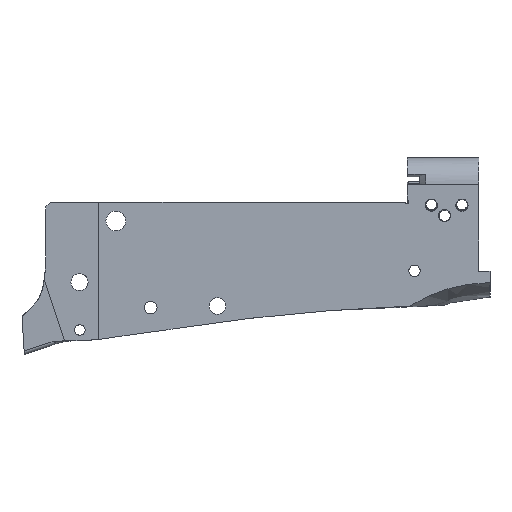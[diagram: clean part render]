
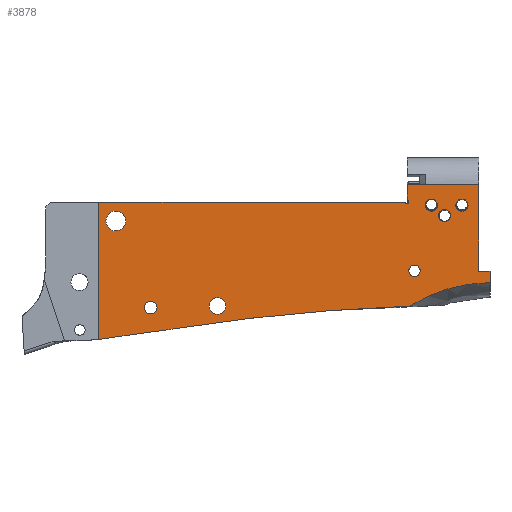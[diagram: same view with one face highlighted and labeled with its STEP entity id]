
A CAD part, left-side view. The second image highlights one B-rep face of the part: STEP entity #3878.
In plain terms, the highlighted planar face has unit normal (-1, 0, 0).
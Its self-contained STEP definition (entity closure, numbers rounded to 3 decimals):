
#116=FACE_BOUND('',#637,.T.);
#117=FACE_BOUND('',#638,.T.);
#118=FACE_BOUND('',#639,.T.);
#119=FACE_BOUND('',#640,.T.);
#120=FACE_BOUND('',#641,.T.);
#121=FACE_BOUND('',#642,.T.);
#122=FACE_BOUND('',#643,.T.);
#223=PLANE('',#4232);
#405=FACE_OUTER_BOUND('',#636,.T.);
#636=EDGE_LOOP('',(#3380,#3381,#3382,#3383,#3384,#3385,#3386,#3387,#3388,
#3389,#3390,#3391,#3392,#3393,#3394));
#637=EDGE_LOOP('',(#3395));
#638=EDGE_LOOP('',(#3396));
#639=EDGE_LOOP('',(#3397));
#640=EDGE_LOOP('',(#3398));
#641=EDGE_LOOP('',(#3399));
#642=EDGE_LOOP('',(#3400));
#643=EDGE_LOOP('',(#3401));
#865=LINE('',#6095,#1246);
#928=LINE('',#6402,#1309);
#962=LINE('',#6740,#1343);
#964=LINE('',#6747,#1345);
#965=LINE('',#6750,#1346);
#992=LINE('',#6824,#1373);
#1018=LINE('',#7119,#1399);
#1023=LINE('',#7130,#1404);
#1246=VECTOR('',#4724,10.);
#1309=VECTOR('',#4911,10.);
#1343=VECTOR('',#5021,10.);
#1345=VECTOR('',#5029,10.);
#1346=VECTOR('',#5034,10.);
#1373=VECTOR('',#5117,10.);
#1399=VECTOR('',#5197,10.);
#1404=VECTOR('',#5210,10.);
#1459=CIRCLE('',#3940,100.);
#1477=CIRCLE('',#3960,827.021);
#1498=CIRCLE('',#3984,600.987);
#1501=CIRCLE('',#3987,45.79);
#1521=CIRCLE('',#4055,1.85);
#1522=CIRCLE('',#4056,1.85);
#1523=CIRCLE('',#4058,1.85);
#1524=CIRCLE('',#4062,2.5);
#1572=CIRCLE('',#4181,3.);
#1573=CIRCLE('',#4184,1.9);
#1587=CIRCLE('',#4231,0.5);
#1588=CIRCLE('',#4233,0.5);
#1589=CIRCLE('',#4234,0.5);
#1590=CIRCLE('',#4235,1.75);
#1601=VERTEX_POINT('',#5389);
#1602=VERTEX_POINT('',#5390);
#1636=VERTEX_POINT('',#5462);
#1667=VERTEX_POINT('',#5531);
#1669=VERTEX_POINT('',#5566);
#1781=VERTEX_POINT('',#5894);
#1783=VERTEX_POINT('',#5967);
#1785=VERTEX_POINT('',#6023);
#1787=VERTEX_POINT('',#6074);
#1792=VERTEX_POINT('',#6092);
#1793=VERTEX_POINT('',#6094);
#1864=VERTEX_POINT('',#6393);
#1867=VERTEX_POINT('',#6400);
#1903=VERTEX_POINT('',#6738);
#1905=VERTEX_POINT('',#6746);
#1909=VERTEX_POINT('',#6767);
#1910=VERTEX_POINT('',#6773);
#1924=VERTEX_POINT('',#6822);
#1942=VERTEX_POINT('',#7124);
#1943=VERTEX_POINT('',#7125);
#1944=VERTEX_POINT('',#7131);
#1945=VERTEX_POINT('',#7134);
#1970=EDGE_CURVE('',#1601,#1602,#1459,.T.);
#2006=EDGE_CURVE('',#1636,#1602,#1477,.T.);
#2042=EDGE_CURVE('',#1601,#1667,#1498,.T.);
#2045=EDGE_CURVE('',#1667,#1669,#1501,.T.);
#2198=EDGE_CURVE('',#1781,#1781,#1521,.T.);
#2201=EDGE_CURVE('',#1783,#1783,#1522,.T.);
#2205=EDGE_CURVE('',#1785,#1785,#1523,.T.);
#2209=EDGE_CURVE('',#1787,#1787,#1524,.T.);
#2219=EDGE_CURVE('',#1792,#1793,#865,.T.);
#2323=EDGE_CURVE('',#1864,#1867,#928,.F.);
#2381=EDGE_CURVE('',#1792,#1903,#962,.T.);
#2384=EDGE_CURVE('',#1793,#1905,#964,.T.);
#2386=EDGE_CURVE('',#1669,#1905,#965,.T.);
#2396=EDGE_CURVE('',#1909,#1909,#1572,.T.);
#2399=EDGE_CURVE('',#1910,#1910,#1573,.T.);
#2423=EDGE_CURVE('',#1924,#1903,#992,.T.);
#2461=EDGE_CURVE('',#1867,#1636,#1018,.T.);
#2464=EDGE_CURVE('',#1942,#1943,#1587,.T.);
#2467=EDGE_CURVE('',#1924,#1943,#1023,.F.);
#2468=EDGE_CURVE('',#1942,#1944,#1588,.T.);
#2469=EDGE_CURVE('',#1864,#1944,#1589,.T.);
#2470=EDGE_CURVE('',#1945,#1945,#1590,.T.);
#3380=ORIENTED_EDGE('',*,*,#1970,.F.);
#3381=ORIENTED_EDGE('',*,*,#2042,.T.);
#3382=ORIENTED_EDGE('',*,*,#2045,.T.);
#3383=ORIENTED_EDGE('',*,*,#2386,.T.);
#3384=ORIENTED_EDGE('',*,*,#2384,.F.);
#3385=ORIENTED_EDGE('',*,*,#2219,.F.);
#3386=ORIENTED_EDGE('',*,*,#2381,.T.);
#3387=ORIENTED_EDGE('',*,*,#2423,.F.);
#3388=ORIENTED_EDGE('',*,*,#2467,.T.);
#3389=ORIENTED_EDGE('',*,*,#2464,.F.);
#3390=ORIENTED_EDGE('',*,*,#2468,.T.);
#3391=ORIENTED_EDGE('',*,*,#2469,.F.);
#3392=ORIENTED_EDGE('',*,*,#2323,.T.);
#3393=ORIENTED_EDGE('',*,*,#2461,.T.);
#3394=ORIENTED_EDGE('',*,*,#2006,.T.);
#3395=ORIENTED_EDGE('',*,*,#2470,.T.);
#3396=ORIENTED_EDGE('',*,*,#2399,.T.);
#3397=ORIENTED_EDGE('',*,*,#2396,.T.);
#3398=ORIENTED_EDGE('',*,*,#2209,.T.);
#3399=ORIENTED_EDGE('',*,*,#2198,.T.);
#3400=ORIENTED_EDGE('',*,*,#2201,.T.);
#3401=ORIENTED_EDGE('',*,*,#2205,.T.);
#3878=ADVANCED_FACE('',(#405,#116,#117,#118,#119,#120,#121,#122),#223,.F.);
#3940=AXIS2_PLACEMENT_3D('',#5391,#4298,#4299);
#3960=AXIS2_PLACEMENT_3D('',#5463,#4356,#4357);
#3984=AXIS2_PLACEMENT_3D('',#5548,#4418,#4419);
#3987=AXIS2_PLACEMENT_3D('',#5568,#4424,#4425);
#4055=AXIS2_PLACEMENT_3D('',#5895,#4686,#4687);
#4056=AXIS2_PLACEMENT_3D('',#5968,#4688,#4689);
#4058=AXIS2_PLACEMENT_3D('',#6025,#4693,#4694);
#4062=AXIS2_PLACEMENT_3D('',#6075,#4703,#4704);
#4181=AXIS2_PLACEMENT_3D('',#6769,#5056,#5057);
#4184=AXIS2_PLACEMENT_3D('',#6775,#5064,#5065);
#4231=AXIS2_PLACEMENT_3D('',#7126,#5204,#5205);
#4232=AXIS2_PLACEMENT_3D('',#7129,#5208,#5209);
#4233=AXIS2_PLACEMENT_3D('',#7132,#5211,#5212);
#4234=AXIS2_PLACEMENT_3D('',#7133,#5213,#5214);
#4235=AXIS2_PLACEMENT_3D('',#7135,#5215,#5216);
#4298=DIRECTION('center_axis',(1.,0.,0.));
#4299=DIRECTION('ref_axis',(0.,-0.143,-0.99));
#4356=DIRECTION('center_axis',(1.,0.,0.));
#4357=DIRECTION('ref_axis',(0.,0.184,0.983));
#4418=DIRECTION('center_axis',(1.,0.,0.));
#4419=DIRECTION('ref_axis',(0.,0.157,0.988));
#4424=DIRECTION('center_axis',(1.,0.,0.));
#4425=DIRECTION('ref_axis',(0.,0.008,1.));
#4686=DIRECTION('center_axis',(1.,0.,0.));
#4687=DIRECTION('ref_axis',(0.,1.,0.));
#4688=DIRECTION('center_axis',(1.,0.,0.));
#4689=DIRECTION('ref_axis',(0.,1.,0.));
#4693=DIRECTION('center_axis',(1.,0.,0.));
#4694=DIRECTION('ref_axis',(0.,-1.,0.));
#4703=DIRECTION('center_axis',(1.,0.,0.));
#4704=DIRECTION('ref_axis',(0.,-1.,0.));
#4724=DIRECTION('',(0.,-1.,0.));
#4911=DIRECTION('',(0.,-1.,0.));
#5021=DIRECTION('',(0.,0.,1.));
#5029=DIRECTION('',(0.,0.,-1.));
#5034=DIRECTION('',(0.,-1.,0.));
#5056=DIRECTION('center_axis',(1.,0.,0.));
#5057=DIRECTION('ref_axis',(0.,1.,0.));
#5064=DIRECTION('center_axis',(1.,0.,0.));
#5065=DIRECTION('ref_axis',(0.,1.,0.));
#5117=DIRECTION('',(0.,-1.,0.));
#5197=DIRECTION('',(0.,0.,-1.));
#5204=DIRECTION('center_axis',(1.,0.,0.));
#5205=DIRECTION('ref_axis',(0.,0.866,-0.5));
#5208=DIRECTION('center_axis',(1.,0.,0.));
#5209=DIRECTION('ref_axis',(0.,1.,0.));
#5210=DIRECTION('',(0.,0.,1.));
#5211=DIRECTION('center_axis',(1.,0.,0.));
#5212=DIRECTION('ref_axis',(0.,1.,0.));
#5213=DIRECTION('center_axis',(1.,0.,0.));
#5214=DIRECTION('ref_axis',(0.,-0.5,0.866));
#5215=DIRECTION('center_axis',(1.,0.,0.));
#5216=DIRECTION('ref_axis',(0.,1.,0.));
#5389=CARTESIAN_POINT('',(-16.48,94.298,-0.025));
#5390=CARTESIAN_POINT('',(-16.48,96.799,-0.385));
#5391=CARTESIAN_POINT('Origin',(-16.48,109.817,98.764));
#5462=CARTESIAN_POINT('',(-16.48,116.868,-3.271));
#5463=CARTESIAN_POINT('Origin',(-16.48,-10.864,-820.368));
#5531=CARTESIAN_POINT('',(-16.48,22.637,6.867));
#5548=CARTESIAN_POINT('Origin',(-16.48,1.034,-593.732));
#5566=CARTESIAN_POINT('',(-16.48,-1.532,13.989));
#5568=CARTESIAN_POINT('Origin',(-16.48,-1.889,-31.8));
#5894=CARTESIAN_POINT('',(-16.48,14.268,37.491));
#5895=CARTESIAN_POINT('Origin',(-16.48,16.118,37.491));
#5967=CARTESIAN_POINT('',(-16.48,4.968,37.491));
#5968=CARTESIAN_POINT('Origin',(-16.48,6.818,37.491));
#6023=CARTESIAN_POINT('',(-16.48,13.918,34.291));
#6025=CARTESIAN_POINT('Origin',(-16.48,12.068,34.291));
#6074=CARTESIAN_POINT('',(-16.48,83.468,6.932));
#6075=CARTESIAN_POINT('Origin',(-16.48,80.968,6.932));
#6092=CARTESIAN_POINT('',(-16.48,1.668,17.422));
#6094=CARTESIAN_POINT('',(-16.48,-1.682,17.422));
#6095=CARTESIAN_POINT('',(-16.48,1.468,17.422));
#6393=CARTESIAN_POINT('',(-16.48,24.334,38.432));
#6400=CARTESIAN_POINT('',(-16.48,116.868,38.432));
#6402=CARTESIAN_POINT('',(-16.48,104.819,38.432));
#6738=CARTESIAN_POINT('',(-16.48,1.668,43.772));
#6740=CARTESIAN_POINT('',(-16.48,1.668,32.945));
#6746=CARTESIAN_POINT('',(-16.48,-1.682,13.989));
#6747=CARTESIAN_POINT('',(-16.48,-1.682,17.922));
#6750=CARTESIAN_POINT('',(-16.48,-1.532,13.989));
#6767=CARTESIAN_POINT('',(-16.48,108.768,32.682));
#6769=CARTESIAN_POINT('Origin',(-16.48,111.768,32.682));
#6773=CARTESIAN_POINT('',(-16.48,99.268,6.432));
#6775=CARTESIAN_POINT('Origin',(-16.48,101.168,6.432));
#6822=CARTESIAN_POINT('',(-16.48,23.468,43.772));
#6824=CARTESIAN_POINT('',(-16.48,23.468,43.772));
#7119=CARTESIAN_POINT('',(-16.48,116.868,9.407));
#7124=CARTESIAN_POINT('',(-16.48,23.218,38.865));
#7125=CARTESIAN_POINT('',(-16.48,23.468,39.298));
#7126=CARTESIAN_POINT('Origin',(-16.48,22.968,39.298));
#7129=CARTESIAN_POINT('Origin',(-16.48,70.369,22.148));
#7130=CARTESIAN_POINT('',(-16.48,23.468,30.29));
#7131=CARTESIAN_POINT('',(-16.48,23.901,38.182));
#7132=CARTESIAN_POINT('Origin',(-16.48,23.468,38.432));
#7133=CARTESIAN_POINT('Origin',(-16.48,24.334,37.932));
#7134=CARTESIAN_POINT('',(-16.48,19.468,17.522));
#7135=CARTESIAN_POINT('Origin',(-16.48,21.218,17.522));
